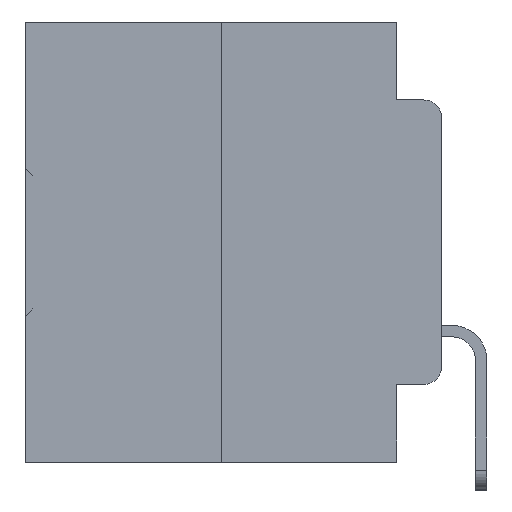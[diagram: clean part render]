
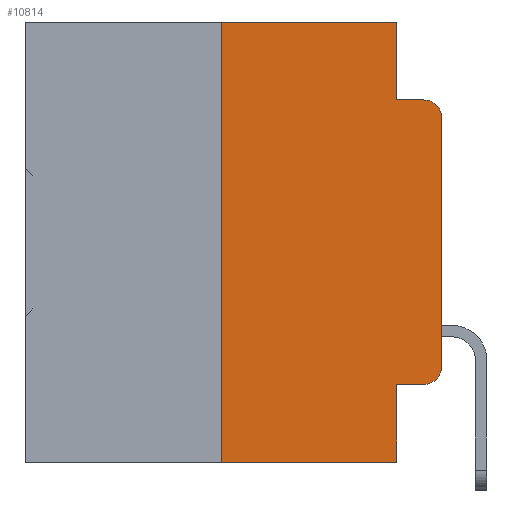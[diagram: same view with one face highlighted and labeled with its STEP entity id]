
A CAD part, left-side view. The second image highlights one B-rep face of the part: STEP entity #10814.
In plain terms, the highlighted planar face has unit normal (-1, 0, 0).
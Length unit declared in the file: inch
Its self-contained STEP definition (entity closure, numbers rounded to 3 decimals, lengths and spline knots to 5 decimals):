
#92 = ORIENTED_EDGE ( 'NONE', *, *, #1086, .F. ) ;
#138 = EDGE_CURVE ( 'NONE', #9409, #13767, #31976, .T. ) ;
#179 = CARTESIAN_POINT ( 'NONE',  ( 0., 0.25, 0. ) ) ;
#345 = LINE ( 'NONE', #1954, #15865 ) ;
#384 = VECTOR ( 'NONE', #12951, 39.37008 ) ;
#400 = DIRECTION ( 'NONE',  ( 0., 0., -1. ) ) ;
#526 = EDGE_CURVE ( 'NONE', #20795, #10424, #18533, .T. ) ;
#712 = LINE ( 'NONE', #11872, #22635 ) ;
#1086 = EDGE_CURVE ( 'NONE', #10424, #14985, #8238, .T. ) ;
#1530 = ORIENTED_EDGE ( 'NONE', *, *, #3345, .T. ) ;
#1954 = CARTESIAN_POINT ( 'NONE',  ( 0., 0., 0. ) ) ;
#2280 = VERTEX_POINT ( 'NONE', #11140 ) ;
#3343 = ORIENTED_EDGE ( 'NONE', *, *, #8054, .T. ) ;
#3345 = EDGE_CURVE ( 'NONE', #29307, #22919, #345, .T. ) ;
#3851 = ORIENTED_EDGE ( 'NONE', *, *, #13835, .F. ) ;
#4093 = DIRECTION ( 'NONE',  ( 0., 0., -1. ) ) ;
#4876 = VERTEX_POINT ( 'NONE', #11526 ) ;
#5467 = DIRECTION ( 'NONE',  ( 0., -1., 0. ) ) ;
#6578 = CARTESIAN_POINT ( 'NONE',  ( 0., 0.02, -0.0885 ) ) ;
#6952 = CARTESIAN_POINT ( 'NONE',  ( 0., 0.051, -0.0885 ) ) ;
#7729 = EDGE_CURVE ( 'NONE', #2280, #20795, #34138, .T. ) ;
#7789 = CARTESIAN_POINT ( 'NONE',  ( 0., 0.25, 0. ) ) ;
#8054 = EDGE_CURVE ( 'NONE', #9409, #4876, #25010, .T. ) ;
#8238 = LINE ( 'NONE', #9273, #384 ) ;
#9005 = AXIS2_PLACEMENT_3D ( 'NONE', #16763, #35444, #19552 ) ;
#9273 = CARTESIAN_POINT ( 'NONE',  ( 0., 0.051, 0. ) ) ;
#9366 = DIRECTION ( 'NONE',  ( 0., -1., 0. ) ) ;
#9409 = VERTEX_POINT ( 'NONE', #16271 ) ;
#9799 = PLANE ( 'NONE',  #25902 ) ;
#9909 = AXIS2_PLACEMENT_3D ( 'NONE', #32781, #16692, #35380 ) ;
#10253 = CARTESIAN_POINT ( 'NONE',  ( 0., 0.473, 0. ) ) ;
#10424 = VERTEX_POINT ( 'NONE', #15490 ) ;
#10814 = ADVANCED_FACE ( 'NONE', ( #27981 ), #9799, .F. ) ;
#11140 = CARTESIAN_POINT ( 'NONE',  ( 0., 0.25, -0.5 ) ) ;
#11211 = CIRCLE ( 'NONE', #9909, 0.02 ) ;
#11526 = CARTESIAN_POINT ( 'NONE',  ( 0., 0.02, -0.4115 ) ) ;
#11872 = CARTESIAN_POINT ( 'NONE',  ( 0., 0.473, -0.5 ) ) ;
#11963 = VECTOR ( 'NONE', #5467, 39.37008 ) ;
#12556 = VECTOR ( 'NONE', #20343, 39.37008 ) ;
#12951 = DIRECTION ( 'NONE',  ( 0., 0., -1. ) ) ;
#13006 = ORIENTED_EDGE ( 'NONE', *, *, #23058, .T. ) ;
#13767 = VERTEX_POINT ( 'NONE', #31459 ) ;
#13835 = EDGE_CURVE ( 'NONE', #14985, #17169, #35935, .T. ) ;
#14985 = VERTEX_POINT ( 'NONE', #17295 ) ;
#15029 = EDGE_CURVE ( 'NONE', #2280, #13767, #712, .T. ) ;
#15490 = CARTESIAN_POINT ( 'NONE',  ( 0., 0.051, 0. ) ) ;
#15865 = VECTOR ( 'NONE', #32606, 39.37008 ) ;
#16271 = CARTESIAN_POINT ( 'NONE',  ( 0., 0.051, -0.4115 ) ) ;
#16692 = DIRECTION ( 'NONE',  ( -1., 0., 0. ) ) ;
#16763 = CARTESIAN_POINT ( 'NONE',  ( 0., 0.02, -0.1085 ) ) ;
#17169 = VERTEX_POINT ( 'NONE', #6578 ) ;
#17295 = CARTESIAN_POINT ( 'NONE',  ( 0., 0.051, -0.0885 ) ) ;
#17404 = ORIENTED_EDGE ( 'NONE', *, *, #138, .F. ) ;
#18533 = LINE ( 'NONE', #10253, #11963 ) ;
#18838 = CARTESIAN_POINT ( 'NONE',  ( 0., 0., -0.1085 ) ) ;
#19339 = CARTESIAN_POINT ( 'NONE',  ( 0., 0., -0.3915 ) ) ;
#19501 = EDGE_CURVE ( 'NONE', #4876, #29307, #11211, .T. ) ;
#19552 = DIRECTION ( 'NONE',  ( 0., 0., -1. ) ) ;
#20343 = DIRECTION ( 'NONE',  ( 0., 0., 1. ) ) ;
#20795 = VERTEX_POINT ( 'NONE', #7789 ) ;
#21160 = DIRECTION ( 'NONE',  ( 1., 0., 0. ) ) ;
#21172 = CARTESIAN_POINT ( 'NONE',  ( 0., 0.051, 0. ) ) ;
#21877 = VECTOR ( 'NONE', #34440, 39.37008 ) ;
#22485 = VECTOR ( 'NONE', #9366, 39.37008 ) ;
#22635 = VECTOR ( 'NONE', #23015, 39.37008 ) ;
#22919 = VERTEX_POINT ( 'NONE', #18838 ) ;
#23015 = DIRECTION ( 'NONE',  ( 0., -1., 0. ) ) ;
#23058 = EDGE_CURVE ( 'NONE', #22919, #17169, #29296, .T. ) ;
#23333 = CARTESIAN_POINT ( 'NONE',  ( 0., 0.051, -0.4115 ) ) ;
#24096 = VECTOR ( 'NONE', #400, 39.37008 ) ;
#25010 = LINE ( 'NONE', #23333, #22485 ) ;
#25902 = AXIS2_PLACEMENT_3D ( 'NONE', #34159, #21160, #4093 ) ;
#27981 = FACE_OUTER_BOUND ( 'NONE', #34578, .T. ) ;
#29124 = ORIENTED_EDGE ( 'NONE', *, *, #19501, .T. ) ;
#29296 = CIRCLE ( 'NONE', #9005, 0.02 ) ;
#29307 = VERTEX_POINT ( 'NONE', #19339 ) ;
#31459 = CARTESIAN_POINT ( 'NONE',  ( 0., 0.051, -0.5 ) ) ;
#31976 = LINE ( 'NONE', #21172, #24096 ) ;
#32606 = DIRECTION ( 'NONE',  ( 0., 0., 1. ) ) ;
#32781 = CARTESIAN_POINT ( 'NONE',  ( 0., 0.02, -0.3915 ) ) ;
#32890 = ORIENTED_EDGE ( 'NONE', *, *, #15029, .T. ) ;
#33306 = ORIENTED_EDGE ( 'NONE', *, *, #7729, .F. ) ;
#34138 = LINE ( 'NONE', #179, #12556 ) ;
#34159 = CARTESIAN_POINT ( 'NONE',  ( 0., 0.473, 0. ) ) ;
#34440 = DIRECTION ( 'NONE',  ( 0., -1., 0. ) ) ;
#34547 = ORIENTED_EDGE ( 'NONE', *, *, #526, .F. ) ;
#34578 = EDGE_LOOP ( 'NONE', ( #1530, #13006, #3851, #92, #34547, #33306, #32890, #17404, #3343, #29124 ) ) ;
#35380 = DIRECTION ( 'NONE',  ( 0., 0., -1. ) ) ;
#35444 = DIRECTION ( 'NONE',  ( -1., 0., 0. ) ) ;
#35935 = LINE ( 'NONE', #6952, #21877 ) ;
